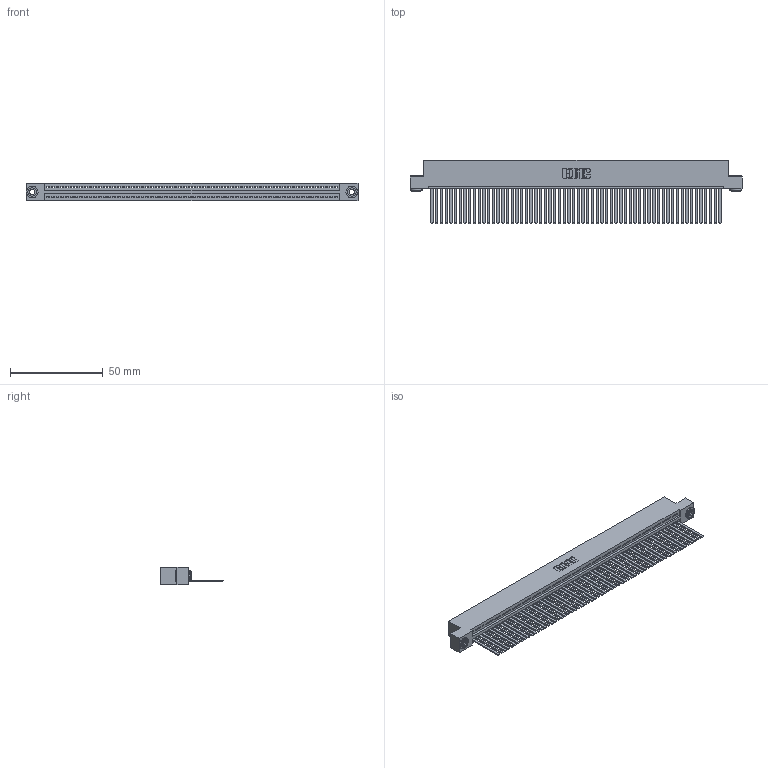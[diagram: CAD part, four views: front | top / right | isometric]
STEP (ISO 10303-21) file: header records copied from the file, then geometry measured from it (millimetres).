
FILE_DESCRIPTION (( 'STEP AP203' ), '1' );
FILE_NAME ('395-062-544-103.STEP', '2019-10-24T19:21:03', ( '' ), ( '' ), 'SwSTEP 2.0', 'SolidWorks 2016', '' );
FILE_SCHEMA (( 'CONFIG_CONTROL_DESIGN' ));
Length unit declared in the file: inch
Products named in the file (4): 345-250-002_345-250-002-102; 395-062-544-103; 345 Part_Flush Mounting Lugs - 0.156 Dia-TH; 345-292-001_345-293-144
Assembly tree (65 placements, depth 2):
  395-062-544-103
    345 Part_Flush Mounting Lugs - 0.156 Dia-TH
    345-292-001_345-293-144  x62
    345-250-002_345-250-002-102  x2
Bounding box: 178.69 x 33.96 x 9.4 mm (x, y, z)
Volume: 17873.3 mm3; surface area: 26394 mm2
Topology: 65 solids, 65 shells, 3388 faces, 10213 edges, 6722 vertices
Faces by surface type: plane 2322, cylinder 1058, cone 8
Entity records: 44436 total; most frequent: CARTESIAN_POINT 7673, ORIENTED_EDGE 7662, DIRECTION 6701, EDGE_CURVE 3831, VECTOR 3431, LINE 3431, VERTEX_POINT 2550, AXIS2_PLACEMENT_3D 1635
